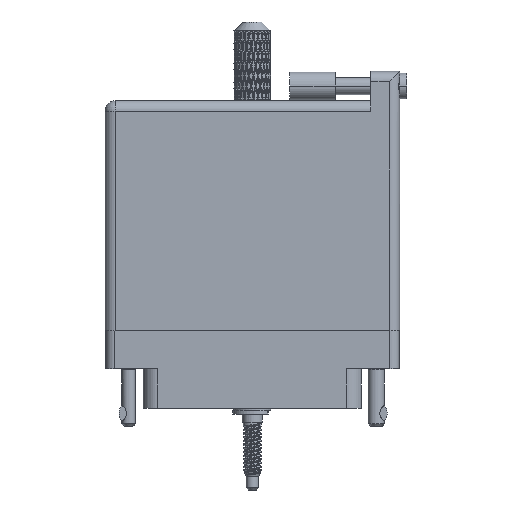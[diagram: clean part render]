
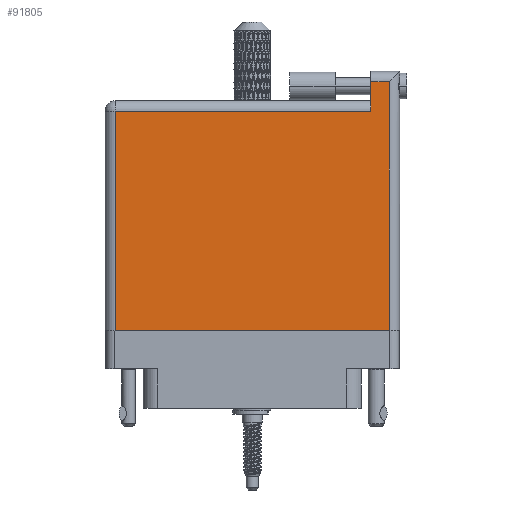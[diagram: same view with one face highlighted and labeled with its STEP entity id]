
A CAD part, front view. The second image highlights one B-rep face of the part: STEP entity #91805.
In plain terms, the highlighted face is planar.
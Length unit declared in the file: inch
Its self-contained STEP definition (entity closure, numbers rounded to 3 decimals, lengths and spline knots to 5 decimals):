
#315 = CARTESIAN_POINT ( 'NONE',  ( 0.07, 0., 0. ) ) ;
#1357 = VECTOR ( 'NONE', #90647, 39.37008 ) ;
#1598 = VECTOR ( 'NONE', #94046, 39.37008 ) ;
#3885 = ORIENTED_EDGE ( 'NONE', *, *, #35881, .T. ) ;
#4326 = LINE ( 'NONE', #6981, #1598 ) ;
#6981 = CARTESIAN_POINT ( 'NONE',  ( 0., 1.696, 0. ) ) ;
#16988 = CARTESIAN_POINT ( 'NONE',  ( 1.938, 0., 0. ) ) ;
#17572 = CARTESIAN_POINT ( 'NONE',  ( 1.811, 1.696, 0. ) ) ;
#19648 = AXIS2_PLACEMENT_3D ( 'NONE', #64417, #46373, #64793 ) ;
#22844 = ORIENTED_EDGE ( 'NONE', *, *, #64261, .T. ) ;
#22990 = CARTESIAN_POINT ( 'NONE',  ( 0., 1.496, 0. ) ) ;
#23699 = VECTOR ( 'NONE', #52191, 39.37008 ) ;
#24083 = CARTESIAN_POINT ( 'NONE',  ( 1.938, 1.696, 0. ) ) ;
#25176 = VERTEX_POINT ( 'NONE', #24083 ) ;
#28436 = EDGE_CURVE ( 'NONE', #48060, #25176, #76152, .T. ) ;
#28697 = VECTOR ( 'NONE', #31269, 39.37008 ) ;
#29437 = VECTOR ( 'NONE', #56823, 39.37008 ) ;
#31269 = DIRECTION ( 'NONE',  ( 0., -1., 0. ) ) ;
#35881 = EDGE_CURVE ( 'NONE', #25176, #44546, #4326, .T. ) ;
#36700 = CARTESIAN_POINT ( 'NONE',  ( 0.07, 1.496, 0. ) ) ;
#44546 = VERTEX_POINT ( 'NONE', #17572 ) ;
#44786 = EDGE_CURVE ( 'NONE', #44546, #73398, #96039, .T. ) ;
#44861 = PLANE ( 'NONE',  #19648 ) ;
#46373 = DIRECTION ( 'NONE',  ( 0., 0., -1. ) ) ;
#48060 = VERTEX_POINT ( 'NONE', #16988 ) ;
#49239 = CARTESIAN_POINT ( 'NONE',  ( 1.811, 1.766, 0. ) ) ;
#52191 = DIRECTION ( 'NONE',  ( 0., -1., 0. ) ) ;
#55685 = CARTESIAN_POINT ( 'NONE',  ( 1.938, 1.766, 0. ) ) ;
#56823 = DIRECTION ( 'NONE',  ( 0., 1., 0. ) ) ;
#64261 = EDGE_CURVE ( 'NONE', #88661, #75606, #66318, .T. ) ;
#64390 = LINE ( 'NONE', #22990, #105681 ) ;
#64417 = CARTESIAN_POINT ( 'NONE',  ( 0., 1.566, 0. ) ) ;
#64793 = DIRECTION ( 'NONE',  ( -1., 0., 0. ) ) ;
#66318 = LINE ( 'NONE', #87550, #23699 ) ;
#71017 = ORIENTED_EDGE ( 'NONE', *, *, #112150, .T. ) ;
#73398 = VERTEX_POINT ( 'NONE', #108555 ) ;
#75606 = VERTEX_POINT ( 'NONE', #315 ) ;
#76152 = LINE ( 'NONE', #55685, #29437 ) ;
#80118 = FACE_OUTER_BOUND ( 'NONE', #90054, .T. ) ;
#82292 = LINE ( 'NONE', #82588, #1357 ) ;
#82588 = CARTESIAN_POINT ( 'NONE',  ( 0., 0., 0. ) ) ;
#83054 = ORIENTED_EDGE ( 'NONE', *, *, #44786, .T. ) ;
#87550 = CARTESIAN_POINT ( 'NONE',  ( 0.07, 0., 0. ) ) ;
#88661 = VERTEX_POINT ( 'NONE', #36700 ) ;
#89412 = ORIENTED_EDGE ( 'NONE', *, *, #28436, .T. ) ;
#90054 = EDGE_LOOP ( 'NONE', ( #71017, #89412, #3885, #83054, #100520, #22844 ) ) ;
#90647 = DIRECTION ( 'NONE',  ( 1., 0., 0. ) ) ;
#91805 = ADVANCED_FACE ( 'NONE', ( #80118 ), #44861, .F. ) ;
#94046 = DIRECTION ( 'NONE',  ( -1., 0., 0. ) ) ;
#96039 = LINE ( 'NONE', #49239, #28697 ) ;
#100520 = ORIENTED_EDGE ( 'NONE', *, *, #112302, .T. ) ;
#100975 = DIRECTION ( 'NONE',  ( -1., 0., 0. ) ) ;
#105681 = VECTOR ( 'NONE', #100975, 39.37008 ) ;
#108555 = CARTESIAN_POINT ( 'NONE',  ( 1.811, 1.496, 0. ) ) ;
#112150 = EDGE_CURVE ( 'NONE', #75606, #48060, #82292, .T. ) ;
#112302 = EDGE_CURVE ( 'NONE', #73398, #88661, #64390, .T. ) ;
